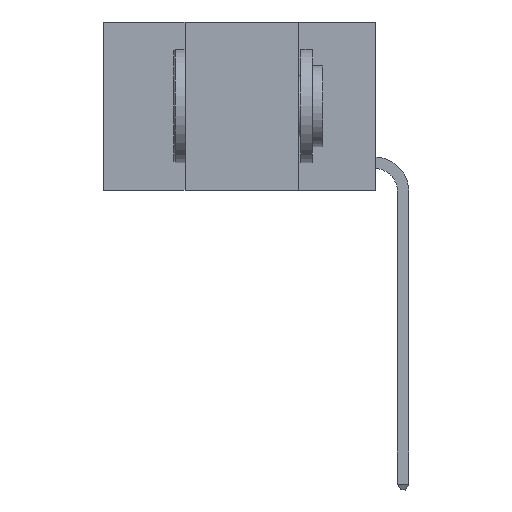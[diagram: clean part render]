
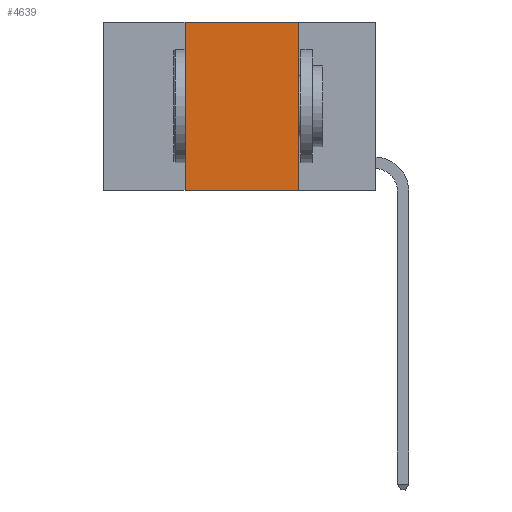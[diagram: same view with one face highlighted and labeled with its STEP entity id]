
A CAD part, left-side view. The second image highlights one B-rep face of the part: STEP entity #4639.
In plain terms, the highlighted planar face has unit normal (-1, 0, 0).
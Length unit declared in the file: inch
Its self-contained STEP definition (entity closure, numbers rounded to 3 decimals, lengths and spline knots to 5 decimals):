
#406 = VERTEX_POINT ( 'NONE', #11601 ) ;
#477 = DIRECTION ( 'NONE',  ( 0., 0., 1. ) ) ;
#868 = DIRECTION ( 'NONE',  ( 0., -1., 0. ) ) ;
#1659 = LINE ( 'NONE', #11797, #8927 ) ;
#2130 = DIRECTION ( 'NONE',  ( 1., 0., 0. ) ) ;
#2525 = VECTOR ( 'NONE', #10684, 39.37008 ) ;
#2836 = LINE ( 'NONE', #3436, #2525 ) ;
#3436 = CARTESIAN_POINT ( 'NONE',  ( 0., 0.17, 0. ) ) ;
#4369 = AXIS2_PLACEMENT_3D ( 'NONE', #8758, #2130, #8797 ) ;
#4474 = DIRECTION ( 'NONE',  ( 0., -1., 0. ) ) ;
#4639 = ADVANCED_FACE ( 'NONE', ( #7864 ), #6079, .F. ) ;
#4701 = ORIENTED_EDGE ( 'NONE', *, *, #7228, .F. ) ;
#5249 = LINE ( 'NONE', #9892, #9709 ) ;
#5508 = CARTESIAN_POINT ( 'NONE',  ( 0., 0.17, -0.37 ) ) ;
#6079 = PLANE ( 'NONE',  #4369 ) ;
#6614 = CARTESIAN_POINT ( 'NONE',  ( 0., 0.17, 0. ) ) ;
#6924 = EDGE_CURVE ( 'NONE', #7238, #8299, #1659, .T. ) ;
#7216 = ORIENTED_EDGE ( 'NONE', *, *, #6924, .F. ) ;
#7228 = EDGE_CURVE ( 'NONE', #8299, #8063, #2836, .T. ) ;
#7238 = VERTEX_POINT ( 'NONE', #11478 ) ;
#7243 = EDGE_CURVE ( 'NONE', #406, #7238, #5249, .T. ) ;
#7245 = EDGE_CURVE ( 'NONE', #406, #8063, #11812, .T. ) ;
#7340 = CARTESIAN_POINT ( 'NONE',  ( 0., 0.6, -0.37 ) ) ;
#7501 = ORIENTED_EDGE ( 'NONE', *, *, #7245, .T. ) ;
#7681 = VECTOR ( 'NONE', #4474, 39.37008 ) ;
#7864 = FACE_OUTER_BOUND ( 'NONE', #10973, .T. ) ;
#8063 = VERTEX_POINT ( 'NONE', #5508 ) ;
#8299 = VERTEX_POINT ( 'NONE', #6614 ) ;
#8758 = CARTESIAN_POINT ( 'NONE',  ( 0., 0.6, 0. ) ) ;
#8797 = DIRECTION ( 'NONE',  ( 0., 0., -1. ) ) ;
#8927 = VECTOR ( 'NONE', #868, 39.37008 ) ;
#9709 = VECTOR ( 'NONE', #477, 39.37008 ) ;
#9892 = CARTESIAN_POINT ( 'NONE',  ( 0., 0.42, 0. ) ) ;
#10684 = DIRECTION ( 'NONE',  ( 0., 0., -1. ) ) ;
#10973 = EDGE_LOOP ( 'NONE', ( #4701, #7216, #11640, #7501 ) ) ;
#11478 = CARTESIAN_POINT ( 'NONE',  ( 0., 0.42, 0. ) ) ;
#11601 = CARTESIAN_POINT ( 'NONE',  ( 0., 0.42, -0.37 ) ) ;
#11640 = ORIENTED_EDGE ( 'NONE', *, *, #7243, .F. ) ;
#11797 = CARTESIAN_POINT ( 'NONE',  ( 0., 0.6, 0. ) ) ;
#11812 = LINE ( 'NONE', #7340, #7681 ) ;
